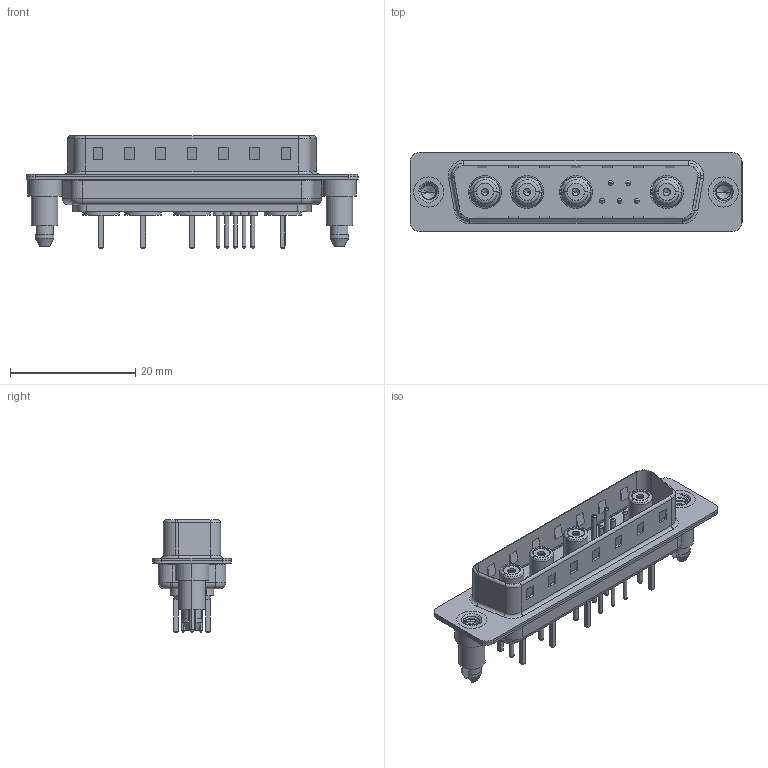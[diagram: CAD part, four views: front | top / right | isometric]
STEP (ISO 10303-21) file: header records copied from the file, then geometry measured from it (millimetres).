
FILE_DESCRIPTION (( 'STEP AP203' ), '1' );
FILE_NAME ('627-9W4-224-7TD.STEP', '2019-06-26T11:53:37', ( '' ), ( '' ), 'SwSTEP 2.0', 'SolidWorks 2016', '' );
FILE_SCHEMA (( 'CONFIG_CONTROL_DESIGN' ));
Length unit declared in the file: millimetre
Products named in the file (14): 627Combo Shell Front_25 Contacts; 627Combo Shell Rear_25 Contacts; 627-9W4-224-7TD; Insulator Socket 2; 627Combo Contact Row 1_24; Insulator Socket; 627Combo Threaded Boardlock_5; 627Combo Contact Row 2_24; Co-Ax Jack_Straight PC Tail; 627Combo Threaded Boardlock_D; Co-Ax Jack Assy_St; 627Combo Housing_9W4; Socket_Str; Locking Collar
Assembly tree (19 placements, depth 3):
  627-9W4-224-7TD
    627Combo Housing_9W4
    627Combo Shell Rear_25 Contacts
    627Combo Shell Front_25 Contacts
    627Combo Threaded Boardlock_D
    Co-Ax Jack Assy_St  x4
      Co-Ax Jack_Straight PC Tail
      Insulator Socket
      Insulator Socket 2
      Locking Collar
      Socket_Str
    627Combo Threaded Boardlock_5
    627Combo Contact Row 1_24  x2
    627Combo Contact Row 2_24  x3
Bounding box: 53 x 12.6 x 17.9 mm (x, y, z)
Volume: 2939.5 mm3; surface area: 8664.3 mm2
Topology: 30 solids, 30 shells, 1063 faces, 2475 edges, 1544 vertices
Faces by surface type: cylinder 435, plane 410, torus 146, cone 49, bspline 15, sphere 8
Entity records: 24703 total; most frequent: CARTESIAN_POINT 7393, DIRECTION 3420, ORIENTED_EDGE 3172, EDGE_CURVE 1586, AXIS2_PLACEMENT_3D 1311, VERTEX_POINT 1004, VECTOR 798, LINE 798
